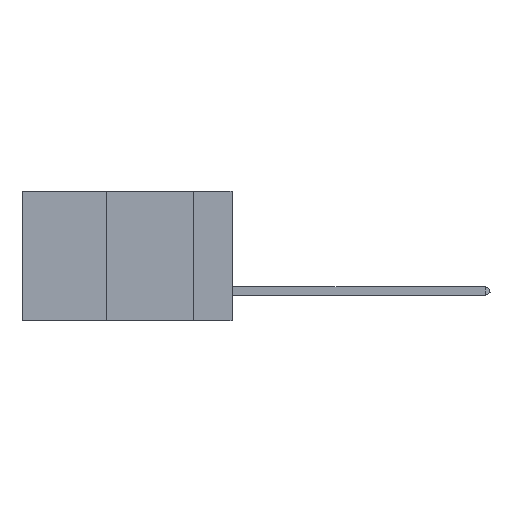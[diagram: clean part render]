
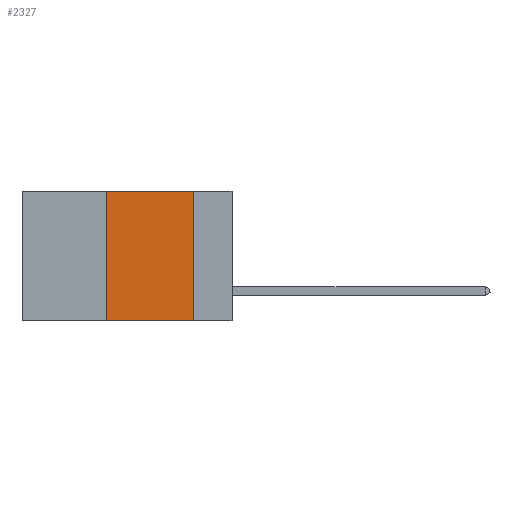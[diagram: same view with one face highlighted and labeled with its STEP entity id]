
A CAD part, left-side view. The second image highlights one B-rep face of the part: STEP entity #2327.
In plain terms, the highlighted planar face has unit normal (-1, 0, 0).
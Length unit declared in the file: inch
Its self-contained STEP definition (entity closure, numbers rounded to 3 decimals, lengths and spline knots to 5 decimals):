
#160 = CARTESIAN_POINT ( 'NONE',  ( 0., 0.11, 0. ) ) ;
#678 = EDGE_CURVE ( 'NONE', #2681, #5049, #3265, .T. ) ;
#702 = DIRECTION ( 'NONE',  ( 0., -1., 0. ) ) ;
#1925 = CARTESIAN_POINT ( 'NONE',  ( 0., 0.36, -0.37 ) ) ;
#2282 = VECTOR ( 'NONE', #702, 39.37008 ) ;
#2327 = ADVANCED_FACE ( 'NONE', ( #3064 ), #5711, .F. ) ;
#2681 = VERTEX_POINT ( 'NONE', #1925 ) ;
#2917 = CARTESIAN_POINT ( 'NONE',  ( 0., 0.36, 0. ) ) ;
#3064 = FACE_OUTER_BOUND ( 'NONE', #10981, .T. ) ;
#3265 = LINE ( 'NONE', #8288, #4206 ) ;
#3418 = ORIENTED_EDGE ( 'NONE', *, *, #7669, .T. ) ;
#3594 = DIRECTION ( 'NONE',  ( 0., 0., -1. ) ) ;
#3771 = DIRECTION ( 'NONE',  ( 1., 0., 0. ) ) ;
#4206 = VECTOR ( 'NONE', #10113, 39.37008 ) ;
#5049 = VERTEX_POINT ( 'NONE', #2917 ) ;
#5246 = DIRECTION ( 'NONE',  ( 0., 0., -1. ) ) ;
#5551 = CARTESIAN_POINT ( 'NONE',  ( 0., 0.6, -0.37 ) ) ;
#5711 = PLANE ( 'NONE',  #6618 ) ;
#6355 = EDGE_CURVE ( 'NONE', #7438, #8287, #7336, .T. ) ;
#6577 = DIRECTION ( 'NONE',  ( 0., -1., 0. ) ) ;
#6618 = AXIS2_PLACEMENT_3D ( 'NONE', #12757, #3771, #3594 ) ;
#6838 = LINE ( 'NONE', #12750, #2282 ) ;
#7336 = LINE ( 'NONE', #160, #7487 ) ;
#7438 = VERTEX_POINT ( 'NONE', #12000 ) ;
#7487 = VECTOR ( 'NONE', #5246, 39.37008 ) ;
#7669 = EDGE_CURVE ( 'NONE', #2681, #8287, #11240, .T. ) ;
#7899 = ORIENTED_EDGE ( 'NONE', *, *, #678, .F. ) ;
#8287 = VERTEX_POINT ( 'NONE', #11598 ) ;
#8288 = CARTESIAN_POINT ( 'NONE',  ( 0., 0.36, 0. ) ) ;
#8418 = EDGE_CURVE ( 'NONE', #5049, #7438, #6838, .T. ) ;
#9359 = VECTOR ( 'NONE', #6577, 39.37008 ) ;
#9769 = ORIENTED_EDGE ( 'NONE', *, *, #8418, .F. ) ;
#10113 = DIRECTION ( 'NONE',  ( 0., 0., 1. ) ) ;
#10981 = EDGE_LOOP ( 'NONE', ( #12199, #9769, #7899, #3418 ) ) ;
#11240 = LINE ( 'NONE', #5551, #9359 ) ;
#11598 = CARTESIAN_POINT ( 'NONE',  ( 0., 0.11, -0.37 ) ) ;
#12000 = CARTESIAN_POINT ( 'NONE',  ( 0., 0.11, 0. ) ) ;
#12199 = ORIENTED_EDGE ( 'NONE', *, *, #6355, .F. ) ;
#12750 = CARTESIAN_POINT ( 'NONE',  ( 0., 0.6, 0. ) ) ;
#12757 = CARTESIAN_POINT ( 'NONE',  ( 0., 0.6, 0. ) ) ;
